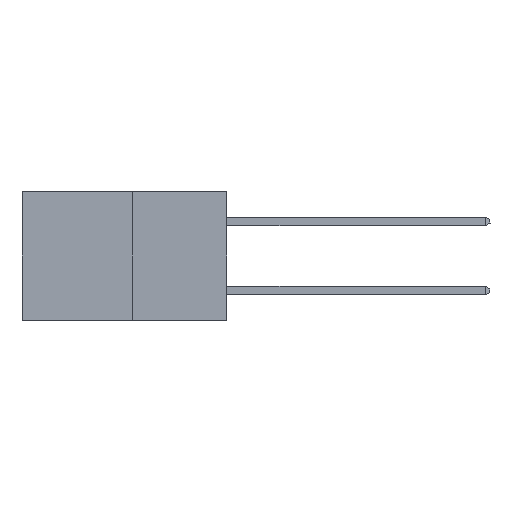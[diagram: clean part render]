
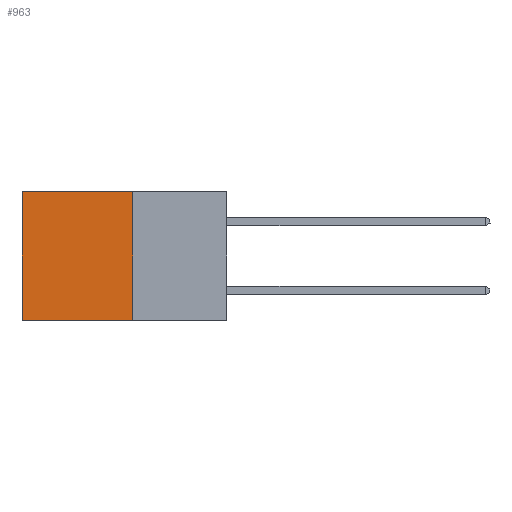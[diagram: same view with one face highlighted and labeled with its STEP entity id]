
A CAD part, left-side view. The second image highlights one B-rep face of the part: STEP entity #963.
In plain terms, the highlighted planar face has unit normal (-1, 0, 0).
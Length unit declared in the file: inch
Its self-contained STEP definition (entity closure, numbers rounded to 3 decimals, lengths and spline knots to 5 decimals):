
#5 = CARTESIAN_POINT ( 'NONE',  ( 0.277, 0.59, 0. ) ) ;
#51 = DIRECTION ( 'NONE',  ( 0., 0., -1. ) ) ;
#58 = DIRECTION ( 'NONE',  ( 1., 0., 0. ) ) ;
#91 = CARTESIAN_POINT ( 'NONE',  ( 0.277, 0.27, -0.37 ) ) ;
#407 = VECTOR ( 'NONE', #16990, 39.37008 ) ;
#963 = ADVANCED_FACE ( 'NONE', ( #13922 ), #17998, .F. ) ;
#2042 = VECTOR ( 'NONE', #7753, 39.37008 ) ;
#2516 = ORIENTED_EDGE ( 'NONE', *, *, #3525, .F. ) ;
#3116 = VECTOR ( 'NONE', #17048, 39.37008 ) ;
#3525 = EDGE_CURVE ( 'NONE', #8092, #7852, #16683, .T. ) ;
#3701 = EDGE_LOOP ( 'NONE', ( #6463, #2516, #10713, #4002 ) ) ;
#3861 = CARTESIAN_POINT ( 'NONE',  ( 0.277, 0.59, -0.37 ) ) ;
#4002 = ORIENTED_EDGE ( 'NONE', *, *, #11262, .T. ) ;
#4405 = CARTESIAN_POINT ( 'NONE',  ( 0.277, 0.27, 0. ) ) ;
#5041 = VECTOR ( 'NONE', #9862, 39.37008 ) ;
#6323 = CARTESIAN_POINT ( 'NONE',  ( 0.277, 0.59, -0.37 ) ) ;
#6463 = ORIENTED_EDGE ( 'NONE', *, *, #15787, .T. ) ;
#7753 = DIRECTION ( 'NONE',  ( 0., 0., -1. ) ) ;
#7852 = VERTEX_POINT ( 'NONE', #3861 ) ;
#8092 = VERTEX_POINT ( 'NONE', #91 ) ;
#9169 = LINE ( 'NONE', #6323, #2042 ) ;
#9665 = CARTESIAN_POINT ( 'NONE',  ( 0.277, 0.27, -0.37 ) ) ;
#9862 = DIRECTION ( 'NONE',  ( 0., 1., 0. ) ) ;
#10289 = CARTESIAN_POINT ( 'NONE',  ( 0.277, 0.27, 0. ) ) ;
#10713 = ORIENTED_EDGE ( 'NONE', *, *, #13085, .F. ) ;
#11262 = EDGE_CURVE ( 'NONE', #11908, #11712, #17596, .T. ) ;
#11712 = VERTEX_POINT ( 'NONE', #5 ) ;
#11734 = AXIS2_PLACEMENT_3D ( 'NONE', #15388, #58, #51 ) ;
#11908 = VERTEX_POINT ( 'NONE', #10289 ) ;
#13085 = EDGE_CURVE ( 'NONE', #11908, #8092, #14930, .T. ) ;
#13922 = FACE_OUTER_BOUND ( 'NONE', #3701, .T. ) ;
#14930 = LINE ( 'NONE', #15580, #407 ) ;
#15388 = CARTESIAN_POINT ( 'NONE',  ( 0.277, 0.27, -0.37 ) ) ;
#15580 = CARTESIAN_POINT ( 'NONE',  ( 0.277, 0.27, -0.37 ) ) ;
#15787 = EDGE_CURVE ( 'NONE', #11712, #7852, #9169, .T. ) ;
#16683 = LINE ( 'NONE', #9665, #5041 ) ;
#16990 = DIRECTION ( 'NONE',  ( 0., 0., -1. ) ) ;
#17048 = DIRECTION ( 'NONE',  ( 0., 1., 0. ) ) ;
#17596 = LINE ( 'NONE', #4405, #3116 ) ;
#17998 = PLANE ( 'NONE',  #11734 ) ;
